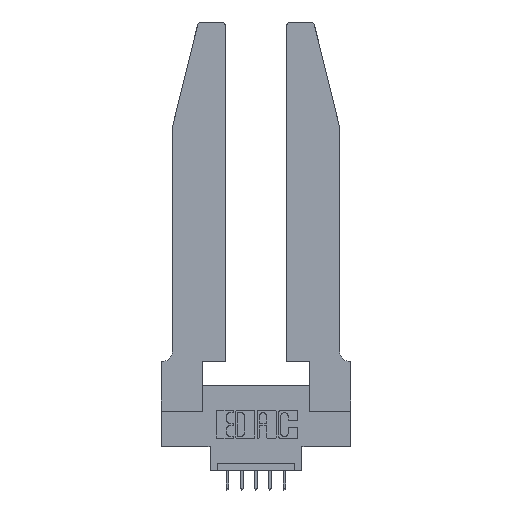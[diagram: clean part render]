
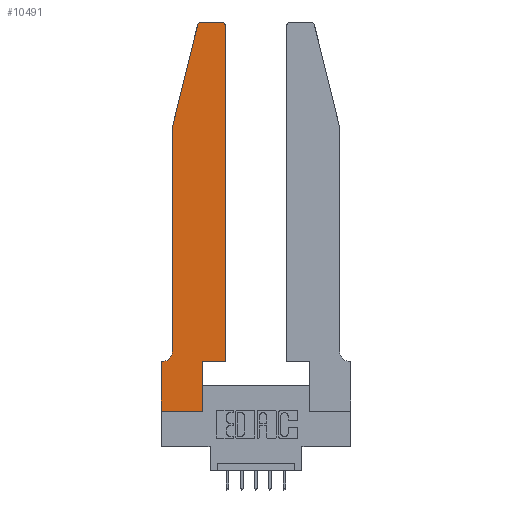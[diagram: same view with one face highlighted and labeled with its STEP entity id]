
A CAD part, top view. The second image highlights one B-rep face of the part: STEP entity #10491.
In plain terms, the highlighted planar face has unit normal (0, 0, 1).
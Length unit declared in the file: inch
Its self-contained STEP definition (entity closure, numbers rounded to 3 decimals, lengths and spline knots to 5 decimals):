
#174 = CARTESIAN_POINT ( 'NONE',  ( 0.4205, 2.75, 0.37 ) ) ;
#297 = CARTESIAN_POINT ( 'NONE',  ( 0.0755, 2., 0.37 ) ) ;
#300 = VECTOR ( 'NONE', #11222, 39.37008 ) ;
#649 = CARTESIAN_POINT ( 'NONE',  ( 0.4505, 0.35, 0.37 ) ) ;
#711 = VERTEX_POINT ( 'NONE', #3694 ) ;
#934 = DIRECTION ( 'NONE',  ( 1., 0., 0. ) ) ;
#1107 = EDGE_CURVE ( 'NONE', #711, #8265, #12446, .T. ) ;
#1219 = VERTEX_POINT ( 'NONE', #174 ) ;
#1264 = DIRECTION ( 'NONE',  ( 1., 0., 0. ) ) ;
#1303 = EDGE_CURVE ( 'NONE', #9350, #13083, #7689, .T. ) ;
#1332 = DIRECTION ( 'NONE',  ( 0., 0., 1. ) ) ;
#1369 = DIRECTION ( 'NONE',  ( -1., 0., 0. ) ) ;
#1528 = LINE ( 'NONE', #5884, #6994 ) ;
#1608 = ORIENTED_EDGE ( 'NONE', *, *, #7377, .T. ) ;
#1674 = CARTESIAN_POINT ( 'NONE',  ( 0., 0.35, 0.37 ) ) ;
#1842 = ORIENTED_EDGE ( 'NONE', *, *, #10662, .T. ) ;
#2226 = EDGE_CURVE ( 'NONE', #6982, #711, #2752, .T. ) ;
#2258 = ORIENTED_EDGE ( 'NONE', *, *, #5513, .T. ) ;
#2746 = EDGE_CURVE ( 'NONE', #1219, #9240, #4705, .T. ) ;
#2752 = LINE ( 'NONE', #4685, #300 ) ;
#2849 = VECTOR ( 'NONE', #934, 39.37008 ) ;
#2944 = DIRECTION ( 'NONE',  ( 1., 0., 0. ) ) ;
#2989 = AXIS2_PLACEMENT_3D ( 'NONE', #5727, #6679, #1369 ) ;
#3415 = CARTESIAN_POINT ( 'NONE',  ( 0., 0., 0.37 ) ) ;
#3451 = EDGE_CURVE ( 'NONE', #8265, #11535, #9686, .T. ) ;
#3525 = EDGE_CURVE ( 'NONE', #11535, #1219, #12932, .T. ) ;
#3548 = CARTESIAN_POINT ( 'NONE',  ( 0., 0.35, 0.37 ) ) ;
#3570 = DIRECTION ( 'NONE',  ( 0., 1., 0. ) ) ;
#3627 = VECTOR ( 'NONE', #7400, 39.37008 ) ;
#3694 = CARTESIAN_POINT ( 'NONE',  ( 0.2865, 0.35, 0.37 ) ) ;
#3702 = AXIS2_PLACEMENT_3D ( 'NONE', #7570, #9493, #4218 ) ;
#3837 = LINE ( 'NONE', #5963, #2849 ) ;
#3921 = ORIENTED_EDGE ( 'NONE', *, *, #10123, .T. ) ;
#4218 = DIRECTION ( 'NONE',  ( 1., 0., 0. ) ) ;
#4242 = EDGE_LOOP ( 'NONE', ( #8568, #3921, #10801, #1842, #2258, #1608, #10909, #8088, #9550, #5997, #9124, #6006 ) ) ;
#4272 = VERTEX_POINT ( 'NONE', #9321 ) ;
#4320 = EDGE_CURVE ( 'NONE', #6131, #12157, #10630, .T. ) ;
#4373 = LINE ( 'NONE', #11668, #10568 ) ;
#4685 = CARTESIAN_POINT ( 'NONE',  ( 0.2865, 0.35, 0.37 ) ) ;
#4705 = LINE ( 'NONE', #6565, #9837 ) ;
#4912 = DIRECTION ( 'NONE',  ( 0., -1., 0. ) ) ;
#5513 = EDGE_CURVE ( 'NONE', #5869, #4272, #11630, .T. ) ;
#5650 = CARTESIAN_POINT ( 'NONE',  ( 0.4505, 2.72, 0.37 ) ) ;
#5727 = CARTESIAN_POINT ( 'NONE',  ( 0.0055, 0.42, 0.37 ) ) ;
#5869 = VERTEX_POINT ( 'NONE', #9122 ) ;
#5884 = CARTESIAN_POINT ( 'NONE',  ( 0.0755, 2., 0.37 ) ) ;
#5963 = CARTESIAN_POINT ( 'NONE',  ( 0., 0., 0.37 ) ) ;
#5997 = ORIENTED_EDGE ( 'NONE', *, *, #1107, .T. ) ;
#6006 = ORIENTED_EDGE ( 'NONE', *, *, #3525, .T. ) ;
#6131 = VERTEX_POINT ( 'NONE', #13405 ) ;
#6565 = CARTESIAN_POINT ( 'NONE',  ( 0.2605, 2.75, 0.37 ) ) ;
#6679 = DIRECTION ( 'NONE',  ( 0., 0., -1. ) ) ;
#6982 = VERTEX_POINT ( 'NONE', #8269 ) ;
#6994 = VECTOR ( 'NONE', #4912, 39.37008 ) ;
#7120 = VECTOR ( 'NONE', #8886, 39.37008 ) ;
#7377 = EDGE_CURVE ( 'NONE', #4272, #9350, #4373, .T. ) ;
#7400 = DIRECTION ( 'NONE',  ( -0.239, -0.971, 0. ) ) ;
#7570 = CARTESIAN_POINT ( 'NONE',  ( 0.284, 2.72, 0.37 ) ) ;
#7689 = LINE ( 'NONE', #13133, #7120 ) ;
#7872 = DIRECTION ( 'NONE',  ( -1., 0., 0. ) ) ;
#7950 = CARTESIAN_POINT ( 'NONE',  ( 0.284, 2.75, 0.37 ) ) ;
#8088 = ORIENTED_EDGE ( 'NONE', *, *, #11965, .T. ) ;
#8265 = VERTEX_POINT ( 'NONE', #11803 ) ;
#8269 = CARTESIAN_POINT ( 'NONE',  ( 0.2865, 0., 0.37 ) ) ;
#8568 = ORIENTED_EDGE ( 'NONE', *, *, #2746, .T. ) ;
#8603 = DIRECTION ( 'NONE',  ( -1., 0., 0. ) ) ;
#8674 = FACE_OUTER_BOUND ( 'NONE', #4242, .T. ) ;
#8886 = DIRECTION ( 'NONE',  ( 0., -1., 0. ) ) ;
#9051 = CARTESIAN_POINT ( 'NONE',  ( 0.4205, 2.72, 0.37 ) ) ;
#9122 = CARTESIAN_POINT ( 'NONE',  ( 0.0755, 0.42, 0.37 ) ) ;
#9124 = ORIENTED_EDGE ( 'NONE', *, *, #3451, .T. ) ;
#9240 = VERTEX_POINT ( 'NONE', #7950 ) ;
#9321 = CARTESIAN_POINT ( 'NONE',  ( 0.0055, 0.35, 0.37 ) ) ;
#9350 = VERTEX_POINT ( 'NONE', #1674 ) ;
#9493 = DIRECTION ( 'NONE',  ( 0., 0., 1. ) ) ;
#9550 = ORIENTED_EDGE ( 'NONE', *, *, #2226, .T. ) ;
#9686 = LINE ( 'NONE', #11903, #9823 ) ;
#9823 = VECTOR ( 'NONE', #3570, 39.37008 ) ;
#9837 = VECTOR ( 'NONE', #7872, 39.37008 ) ;
#10123 = EDGE_CURVE ( 'NONE', #9240, #6131, #13464, .T. ) ;
#10142 = AXIS2_PLACEMENT_3D ( 'NONE', #3548, #1332, #1264 ) ;
#10491 = ADVANCED_FACE ( 'NONE', ( #8674 ), #13066, .T. ) ;
#10568 = VECTOR ( 'NONE', #8603, 39.37008 ) ;
#10630 = LINE ( 'NONE', #11531, #3627 ) ;
#10662 = EDGE_CURVE ( 'NONE', #12157, #5869, #1528, .T. ) ;
#10801 = ORIENTED_EDGE ( 'NONE', *, *, #4320, .T. ) ;
#10909 = ORIENTED_EDGE ( 'NONE', *, *, #1303, .T. ) ;
#10929 = AXIS2_PLACEMENT_3D ( 'NONE', #9051, #13227, #11076 ) ;
#11076 = DIRECTION ( 'NONE',  ( 1., 0., 0. ) ) ;
#11222 = DIRECTION ( 'NONE',  ( 0., 1., 0. ) ) ;
#11531 = CARTESIAN_POINT ( 'NONE',  ( 0.0755, 2., 0.37 ) ) ;
#11535 = VERTEX_POINT ( 'NONE', #5650 ) ;
#11630 = CIRCLE ( 'NONE', #2989, 0.07 ) ;
#11668 = CARTESIAN_POINT ( 'NONE',  ( 0.0755, 0.35, 0.37 ) ) ;
#11803 = CARTESIAN_POINT ( 'NONE',  ( 0.4505, 0.35, 0.37 ) ) ;
#11903 = CARTESIAN_POINT ( 'NONE',  ( 0.4505, 0.35, 0.37 ) ) ;
#11965 = EDGE_CURVE ( 'NONE', #13083, #6982, #3837, .T. ) ;
#12157 = VERTEX_POINT ( 'NONE', #297 ) ;
#12229 = VECTOR ( 'NONE', #2944, 39.37008 ) ;
#12446 = LINE ( 'NONE', #649, #12229 ) ;
#12932 = CIRCLE ( 'NONE', #10929, 0.03 ) ;
#13066 = PLANE ( 'NONE',  #10142 ) ;
#13083 = VERTEX_POINT ( 'NONE', #3415 ) ;
#13133 = CARTESIAN_POINT ( 'NONE',  ( 0., 0., 0.37 ) ) ;
#13227 = DIRECTION ( 'NONE',  ( 0., 0., 1. ) ) ;
#13405 = CARTESIAN_POINT ( 'NONE',  ( 0.25487, 2.72718, 0.37 ) ) ;
#13464 = CIRCLE ( 'NONE', #3702, 0.03 ) ;
